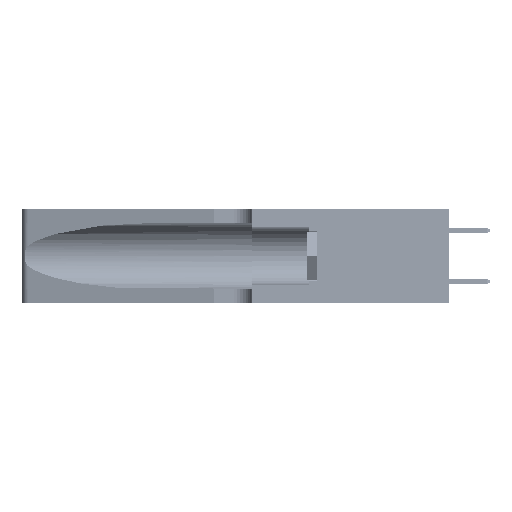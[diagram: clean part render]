
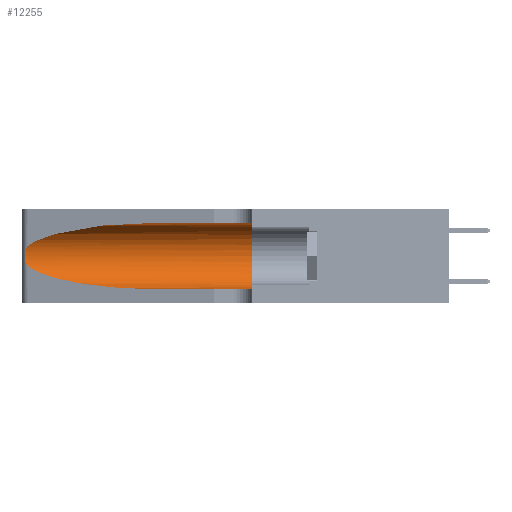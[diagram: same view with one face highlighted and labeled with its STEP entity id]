
A CAD part, left-side view. The second image highlights one B-rep face of the part: STEP entity #12255.
In plain terms, the highlighted cylindrical face has radius 3.308 mm (diameter 6.617 mm), a partial arc.
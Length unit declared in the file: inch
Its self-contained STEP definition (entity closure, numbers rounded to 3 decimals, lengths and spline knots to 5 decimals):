
#263 = DIRECTION ( 'NONE',  ( 0., 0., 1. ) ) ;
#1538 = LINE ( 'NONE', #43440, #34919 ) ;
#1612 = CARTESIAN_POINT ( 'NONE',  ( 0.25487, 1.22718, 0.22369 ) ) ;
#2532 = CIRCLE ( 'NONE', #24417, 0.13025 ) ;
#2681 = CARTESIAN_POINT ( 'NONE',  ( 0.25639, 1.23184, 0.21858 ) ) ;
#4053 = ORIENTED_EDGE ( 'NONE', *, *, #6555, .T. ) ;
#4282 = CARTESIAN_POINT ( 'NONE',  ( 0.1305, 0.35, 0.185 ) ) ;
#6199 = CARTESIAN_POINT ( 'NONE',  ( 0.25487, 1.22718, 0.14631 ) ) ;
#6555 = EDGE_CURVE ( 'NONE', #38113, #36949, #48572, .T. ) ;
#6563 = EDGE_CURVE ( 'NONE', #49405, #18087, #39557, .T. ) ;
#6709 = CARTESIAN_POINT ( 'NONE',  ( 0.25555, 1.22993, 0.14849 ) ) ;
#7077 = EDGE_CURVE ( 'NONE', #49405, #40442, #44940, .T. ) ;
#8546 = VERTEX_POINT ( 'NONE', #25661 ) ;
#9644 = VECTOR ( 'NONE', #43860, 39.37008 ) ;
#9769 = EDGE_CURVE ( 'NONE', #36949, #8546, #1538, .T. ) ;
#10953 = DIRECTION ( 'NONE',  ( 0., 0., -1. ) ) ;
#12255 = ADVANCED_FACE ( 'NONE', ( #33271 ), #29601, .F. ) ;
#12936 = DIRECTION ( 'NONE',  ( 0., -1., 0. ) ) ;
#14019 = CARTESIAN_POINT ( 'NONE',  ( 0.25854, 1.2359, 0.20912 ) ) ;
#14186 = CARTESIAN_POINT ( 'NONE',  ( 0.25856, 1.23593, 0.16098 ) ) ;
#14357 = CARTESIAN_POINT ( 'NONE',  ( 0.26018, 1.23835, 0.19895 ) ) ;
#15790 = CARTESIAN_POINT ( 'NONE',  ( 0.25487, 1.22718, 0.22369 ) ) ;
#16211 = EDGE_CURVE ( 'NONE', #40442, #8546, #2532, .T. ) ;
#16394 = CARTESIAN_POINT ( 'NONE',  ( 0.25487, 1.22718, 0.14631 ) ) ;
#16938 = CARTESIAN_POINT ( 'NONE',  ( 0.1305, 1.61858, 0.31525 ) ) ;
#17583 = CARTESIAN_POINT ( 'NONE',  ( 0.26017, 1.23833, 0.17102 ) ) ;
#17751 = CARTESIAN_POINT ( 'NONE',  ( 0.25487, 1.22718, 0.22369 ) ) ;
#18053 = ORIENTED_EDGE ( 'NONE', *, *, #6563, .T. ) ;
#18087 = VERTEX_POINT ( 'NONE', #15790 ) ;
#18591 = B_SPLINE_CURVE_WITH_KNOTS ( 'NONE', 3,
 ( #17751, #41597, #2681, #49064, #14019, #14357, #44991, #25604, #17583, #14186, #45324, #37847, #6709, #6199 ),
 .UNSPECIFIED., .F., .F.,
 ( 4, 2, 2, 2, 2, 2, 4 ),
 ( 0., 0.00027, 0.00053, 0.00107, 0.0016, 0.00187, 0.00214 ),
 .UNSPECIFIED. ) ;
#21381 = CARTESIAN_POINT ( 'NONE',  ( 0.25487, 1.22718, 0.14631 ) ) ;
#23954 = AXIS2_PLACEMENT_3D ( 'NONE', #41608, #26282, #10953 ) ;
#24417 = AXIS2_PLACEMENT_3D ( 'NONE', #4282, #43079, #263 ) ;
#25204 = CARTESIAN_POINT ( 'NONE',  ( 0.1305, 0.72297, 0.05475 ) ) ;
#25604 = CARTESIAN_POINT ( 'NONE',  ( 0.26075, 1.23896, 0.178 ) ) ;
#25661 = CARTESIAN_POINT ( 'NONE',  ( 0.1305, 0.35, 0.05475 ) ) ;
#26282 = DIRECTION ( 'NONE',  ( 0., -1., 0. ) ) ;
#26781 = ORIENTED_EDGE ( 'NONE', *, *, #16211, .F. ) ;
#29418 = CARTESIAN_POINT ( 'NONE',  ( 0.2373, 1.15595, 0.28018 ) ) ;
#29529 = ORIENTED_EDGE ( 'NONE', *, *, #40206, .T. ) ;
#29601 = CYLINDRICAL_SURFACE ( 'NONE', #23954, 0.13025 ) ;
#31447 = ORIENTED_EDGE ( 'NONE', *, *, #7077, .F. ) ;
#33164 = CARTESIAN_POINT ( 'NONE',  ( 0.1305, 0.72297, 0.05475 ) ) ;
#33271 = FACE_OUTER_BOUND ( 'NONE', #37190, .T. ) ;
#34919 = VECTOR ( 'NONE', #12936, 39.37008 ) ;
#35391 = ORIENTED_EDGE ( 'NONE', *, *, #9769, .T. ) ;
#36949 = VERTEX_POINT ( 'NONE', #25204 ) ;
#37081 = CARTESIAN_POINT ( 'NONE',  ( 0.18966, 0.96281, 0.31525 ) ) ;
#37190 = EDGE_LOOP ( 'NONE', ( #18053, #29529, #4053, #35391, #26781, #31447 ) ) ;
#37245 = CARTESIAN_POINT ( 'NONE',  ( 0.18966, 0.96281, 0.05475 ) ) ;
#37847 = CARTESIAN_POINT ( 'NONE',  ( 0.25639, 1.23186, 0.15144 ) ) ;
#38113 = VERTEX_POINT ( 'NONE', #16394 ) ;
#39557 =( BOUNDED_CURVE ( )  B_SPLINE_CURVE ( 3, ( #40676, #37081, #29418, #1612 ),
 .UNSPECIFIED., .F., .F. ) 
 B_SPLINE_CURVE_WITH_KNOTS ( ( 4, 4 ),
 ( 1.5708, 2.84003 ),
 .UNSPECIFIED. ) 
 CURVE ( )  GEOMETRIC_REPRESENTATION_ITEM ( )  RATIONAL_B_SPLINE_CURVE ( ( 1., 0.87, 0.87, 1. ) ) 
 REPRESENTATION_ITEM ( '' )  );
#40206 = EDGE_CURVE ( 'NONE', #18087, #38113, #18591, .T. ) ;
#40442 = VERTEX_POINT ( 'NONE', #46661 ) ;
#40676 = CARTESIAN_POINT ( 'NONE',  ( 0.1305, 0.72297, 0.31525 ) ) ;
#41597 = CARTESIAN_POINT ( 'NONE',  ( 0.25555, 1.22994, 0.2215 ) ) ;
#41608 = CARTESIAN_POINT ( 'NONE',  ( 0.1305, 1.61858, 0.185 ) ) ;
#43079 = DIRECTION ( 'NONE',  ( 0., 1., 0. ) ) ;
#43440 = CARTESIAN_POINT ( 'NONE',  ( 0.1305, 1.61858, 0.05475 ) ) ;
#43860 = DIRECTION ( 'NONE',  ( 0., -1., 0. ) ) ;
#44728 = CARTESIAN_POINT ( 'NONE',  ( 0.2373, 1.15595, 0.08982 ) ) ;
#44940 = LINE ( 'NONE', #16938, #9644 ) ;
#44991 = CARTESIAN_POINT ( 'NONE',  ( 0.26075, 1.23896, 0.19203 ) ) ;
#45324 = CARTESIAN_POINT ( 'NONE',  ( 0.25789, 1.23486, 0.15765 ) ) ;
#46661 = CARTESIAN_POINT ( 'NONE',  ( 0.1305, 0.35, 0.31525 ) ) ;
#47561 = CARTESIAN_POINT ( 'NONE',  ( 0.1305, 0.72297, 0.31525 ) ) ;
#48572 =( BOUNDED_CURVE ( )  B_SPLINE_CURVE ( 3, ( #21381, #44728, #37245, #33164 ),
 .UNSPECIFIED., .F., .F. ) 
 B_SPLINE_CURVE_WITH_KNOTS ( ( 4, 4 ),
 ( 3.44316, 4.71239 ),
 .UNSPECIFIED. ) 
 CURVE ( )  GEOMETRIC_REPRESENTATION_ITEM ( )  RATIONAL_B_SPLINE_CURVE ( ( 1., 0.87, 0.87, 1. ) ) 
 REPRESENTATION_ITEM ( '' )  );
#49064 = CARTESIAN_POINT ( 'NONE',  ( 0.25787, 1.23484, 0.2124 ) ) ;
#49405 = VERTEX_POINT ( 'NONE', #47561 ) ;
